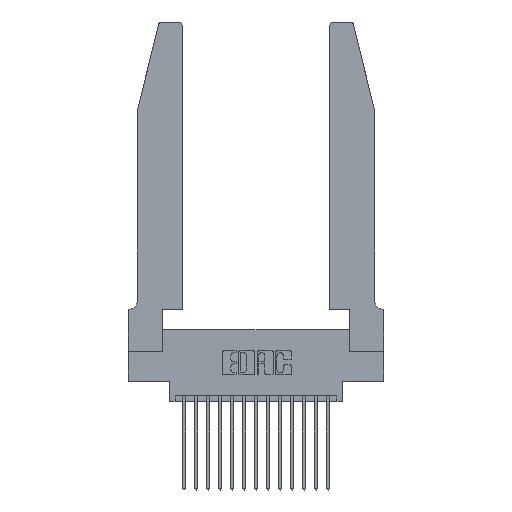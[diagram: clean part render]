
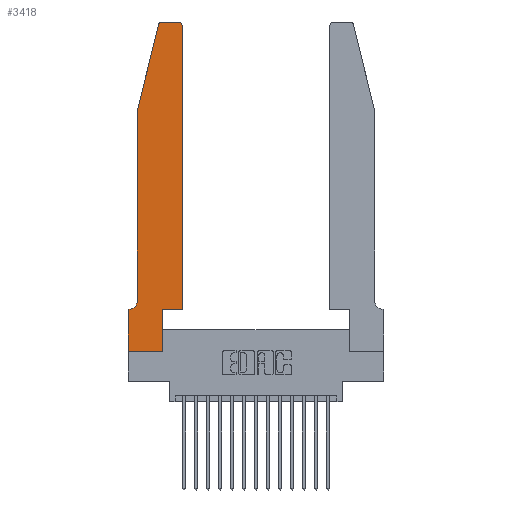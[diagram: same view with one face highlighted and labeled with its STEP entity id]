
A CAD part, top view. The second image highlights one B-rep face of the part: STEP entity #3418.
In plain terms, the highlighted planar face has unit normal (0, 0, 1).
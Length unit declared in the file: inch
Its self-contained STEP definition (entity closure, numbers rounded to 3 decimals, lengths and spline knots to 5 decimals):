
#39 = CARTESIAN_POINT ( 'NONE',  ( 0.284, 2.72, 0.37 ) ) ;
#106 = VECTOR ( 'NONE', #2919, 39.37008 ) ;
#516 = ORIENTED_EDGE ( 'NONE', *, *, #12746, .T. ) ;
#531 = EDGE_CURVE ( 'NONE', #1040, #17234, #7680, .T. ) ;
#541 = DIRECTION ( 'NONE',  ( -1., 0., 0. ) ) ;
#668 = ORIENTED_EDGE ( 'NONE', *, *, #10120, .T. ) ;
#760 = LINE ( 'NONE', #10577, #15506 ) ;
#1040 = VERTEX_POINT ( 'NONE', #3948 ) ;
#1069 = ORIENTED_EDGE ( 'NONE', *, *, #1943, .T. ) ;
#1624 = DIRECTION ( 'NONE',  ( 1., 0., 0. ) ) ;
#1691 = CARTESIAN_POINT ( 'NONE',  ( 0.4505, 2.72, 0.37 ) ) ;
#1923 = CARTESIAN_POINT ( 'NONE',  ( 0.0755, 2., 0.37 ) ) ;
#1943 = EDGE_CURVE ( 'NONE', #9125, #14626, #13741, .T. ) ;
#2500 = CARTESIAN_POINT ( 'NONE',  ( 0.4505, 0.35, 0.37 ) ) ;
#2593 = CARTESIAN_POINT ( 'NONE',  ( 0., 0., 0.37 ) ) ;
#2615 = CIRCLE ( 'NONE', #3575, 0.03 ) ;
#2835 = CARTESIAN_POINT ( 'NONE',  ( 0., 0., 0.37 ) ) ;
#2914 = DIRECTION ( 'NONE',  ( 0., 0., 1. ) ) ;
#2919 = DIRECTION ( 'NONE',  ( 0., -1., 0. ) ) ;
#2960 = DIRECTION ( 'NONE',  ( 1., 0., 0. ) ) ;
#3079 = CIRCLE ( 'NONE', #3919, 0.07 ) ;
#3232 = ORIENTED_EDGE ( 'NONE', *, *, #18024, .T. ) ;
#3240 = DIRECTION ( 'NONE',  ( 1., 0., 0. ) ) ;
#3418 = ADVANCED_FACE ( 'NONE', ( #14598 ), #12724, .T. ) ;
#3508 = CARTESIAN_POINT ( 'NONE',  ( 0.25487, 2.72718, 0.37 ) ) ;
#3575 = AXIS2_PLACEMENT_3D ( 'NONE', #39, #10531, #1624 ) ;
#3673 = VERTEX_POINT ( 'NONE', #8896 ) ;
#3919 = AXIS2_PLACEMENT_3D ( 'NONE', #16403, #7749, #17822 ) ;
#3948 = CARTESIAN_POINT ( 'NONE',  ( 0., 0.35, 0.37 ) ) ;
#4221 = DIRECTION ( 'NONE',  ( 0., 0., 1. ) ) ;
#4386 = CARTESIAN_POINT ( 'NONE',  ( 0.4505, 0.35, 0.37 ) ) ;
#4430 = AXIS2_PLACEMENT_3D ( 'NONE', #4485, #2914, #2960 ) ;
#4485 = CARTESIAN_POINT ( 'NONE',  ( 0., 0.35, 0.37 ) ) ;
#4777 = EDGE_LOOP ( 'NONE', ( #5008, #5327, #18559, #516, #6536, #16329, #13113, #668, #9191, #1069, #6414, #3232 ) ) ;
#5008 = ORIENTED_EDGE ( 'NONE', *, *, #8799, .T. ) ;
#5327 = ORIENTED_EDGE ( 'NONE', *, *, #7648, .T. ) ;
#5623 = DIRECTION ( 'NONE',  ( -0.239, -0.971, 0. ) ) ;
#6414 = ORIENTED_EDGE ( 'NONE', *, *, #7513, .T. ) ;
#6536 = ORIENTED_EDGE ( 'NONE', *, *, #16256, .T. ) ;
#6932 = AXIS2_PLACEMENT_3D ( 'NONE', #12977, #4221, #14390 ) ;
#7168 = VERTEX_POINT ( 'NONE', #9381 ) ;
#7176 = CARTESIAN_POINT ( 'NONE',  ( 0.284, 2.75, 0.37 ) ) ;
#7352 = VERTEX_POINT ( 'NONE', #8485 ) ;
#7513 = EDGE_CURVE ( 'NONE', #14626, #15551, #12300, .T. ) ;
#7648 = EDGE_CURVE ( 'NONE', #16645, #15651, #2615, .T. ) ;
#7680 = LINE ( 'NONE', #2835, #106 ) ;
#7749 = DIRECTION ( 'NONE',  ( 0., 0., -1. ) ) ;
#7900 = VECTOR ( 'NONE', #5623, 39.37008 ) ;
#7946 = VECTOR ( 'NONE', #11689, 39.37008 ) ;
#8327 = CARTESIAN_POINT ( 'NONE',  ( 0.2865, 0., 0.37 ) ) ;
#8416 = VERTEX_POINT ( 'NONE', #1923 ) ;
#8485 = CARTESIAN_POINT ( 'NONE',  ( 0.0755, 0.42, 0.37 ) ) ;
#8799 = EDGE_CURVE ( 'NONE', #7168, #16645, #17815, .T. ) ;
#8896 = CARTESIAN_POINT ( 'NONE',  ( 0.0055, 0.35, 0.37 ) ) ;
#9030 = EDGE_CURVE ( 'NONE', #3673, #1040, #13783, .T. ) ;
#9125 = VERTEX_POINT ( 'NONE', #13919 ) ;
#9191 = ORIENTED_EDGE ( 'NONE', *, *, #13143, .T. ) ;
#9381 = CARTESIAN_POINT ( 'NONE',  ( 0.4205, 2.75, 0.37 ) ) ;
#10120 = EDGE_CURVE ( 'NONE', #17234, #10684, #18661, .T. ) ;
#10531 = DIRECTION ( 'NONE',  ( 0., 0., 1. ) ) ;
#10577 = CARTESIAN_POINT ( 'NONE',  ( 0.2865, 0.35, 0.37 ) ) ;
#10684 = VERTEX_POINT ( 'NONE', #8327 ) ;
#10888 = LINE ( 'NONE', #14310, #7900 ) ;
#11070 = VECTOR ( 'NONE', #17233, 39.37008 ) ;
#11276 = VECTOR ( 'NONE', #18136, 39.37008 ) ;
#11689 = DIRECTION ( 'NONE',  ( 0., 1., 0. ) ) ;
#12053 = DIRECTION ( 'NONE',  ( 0., 1., 0. ) ) ;
#12300 = LINE ( 'NONE', #4386, #7946 ) ;
#12724 = PLANE ( 'NONE',  #4430 ) ;
#12746 = EDGE_CURVE ( 'NONE', #8416, #7352, #18410, .T. ) ;
#12877 = VECTOR ( 'NONE', #3240, 39.37008 ) ;
#12977 = CARTESIAN_POINT ( 'NONE',  ( 0.4205, 2.72, 0.37 ) ) ;
#13004 = CARTESIAN_POINT ( 'NONE',  ( 0., 0., 0.37 ) ) ;
#13113 = ORIENTED_EDGE ( 'NONE', *, *, #531, .T. ) ;
#13143 = EDGE_CURVE ( 'NONE', #10684, #9125, #760, .T. ) ;
#13353 = VECTOR ( 'NONE', #541, 39.37008 ) ;
#13569 = VECTOR ( 'NONE', #18877, 39.37008 ) ;
#13741 = LINE ( 'NONE', #2500, #12877 ) ;
#13783 = LINE ( 'NONE', #16688, #13353 ) ;
#13919 = CARTESIAN_POINT ( 'NONE',  ( 0.2865, 0.35, 0.37 ) ) ;
#14080 = CIRCLE ( 'NONE', #6932, 0.03 ) ;
#14310 = CARTESIAN_POINT ( 'NONE',  ( 0.0755, 2., 0.37 ) ) ;
#14390 = DIRECTION ( 'NONE',  ( 1., 0., 0. ) ) ;
#14598 = FACE_OUTER_BOUND ( 'NONE', #4777, .T. ) ;
#14626 = VERTEX_POINT ( 'NONE', #15667 ) ;
#15506 = VECTOR ( 'NONE', #12053, 39.37008 ) ;
#15551 = VERTEX_POINT ( 'NONE', #1691 ) ;
#15651 = VERTEX_POINT ( 'NONE', #3508 ) ;
#15667 = CARTESIAN_POINT ( 'NONE',  ( 0.4505, 0.35, 0.37 ) ) ;
#16256 = EDGE_CURVE ( 'NONE', #7352, #3673, #3079, .T. ) ;
#16329 = ORIENTED_EDGE ( 'NONE', *, *, #9030, .T. ) ;
#16403 = CARTESIAN_POINT ( 'NONE',  ( 0.0055, 0.42, 0.37 ) ) ;
#16603 = EDGE_CURVE ( 'NONE', #15651, #8416, #10888, .T. ) ;
#16645 = VERTEX_POINT ( 'NONE', #7176 ) ;
#16688 = CARTESIAN_POINT ( 'NONE',  ( 0.0755, 0.35, 0.37 ) ) ;
#16731 = CARTESIAN_POINT ( 'NONE',  ( 0.0755, 2., 0.37 ) ) ;
#17233 = DIRECTION ( 'NONE',  ( 1., 0., 0. ) ) ;
#17234 = VERTEX_POINT ( 'NONE', #13004 ) ;
#17434 = CARTESIAN_POINT ( 'NONE',  ( 0.2605, 2.75, 0.37 ) ) ;
#17815 = LINE ( 'NONE', #17434, #13569 ) ;
#17822 = DIRECTION ( 'NONE',  ( -1., 0., 0. ) ) ;
#18024 = EDGE_CURVE ( 'NONE', #15551, #7168, #14080, .T. ) ;
#18136 = DIRECTION ( 'NONE',  ( 0., -1., 0. ) ) ;
#18410 = LINE ( 'NONE', #16731, #11276 ) ;
#18559 = ORIENTED_EDGE ( 'NONE', *, *, #16603, .T. ) ;
#18661 = LINE ( 'NONE', #2593, #11070 ) ;
#18877 = DIRECTION ( 'NONE',  ( -1., 0., 0. ) ) ;
